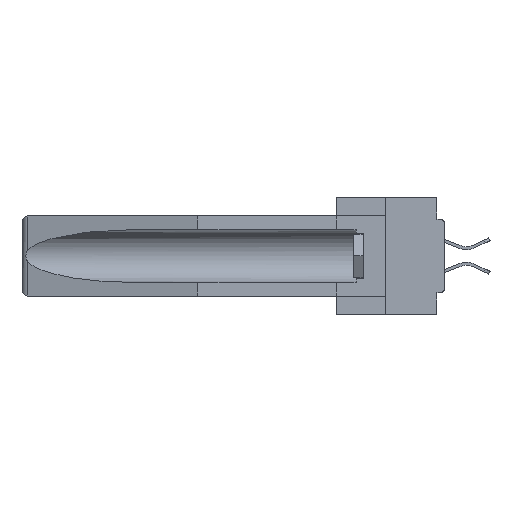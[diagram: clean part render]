
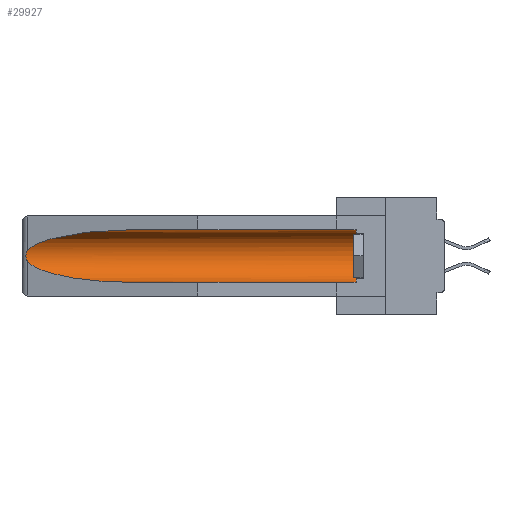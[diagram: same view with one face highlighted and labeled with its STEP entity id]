
A CAD part, left-side view. The second image highlights one B-rep face of the part: STEP entity #29927.
In plain terms, the highlighted cylindrical face has radius 2.857 mm (diameter 5.715 mm), a partial arc.
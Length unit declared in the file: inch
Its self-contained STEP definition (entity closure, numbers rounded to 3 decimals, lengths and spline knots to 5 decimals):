
#23 = DIRECTION ( 'NONE',  ( 0., 1., 0. ) ) ;
#1251 = CARTESIAN_POINT ( 'NONE',  ( 0.26537, 1.52718, -0.19328 ) ) ;
#2004 = CARTESIAN_POINT ( 'NONE',  ( 0.2673, 1.5327, -0.16383 ) ) ;
#4246 = AXIS2_PLACEMENT_3D ( 'NONE', #12824, #24051, #27007 ) ;
#5153 = EDGE_CURVE ( 'NONE', #10641, #20374, #31416, .T. ) ;
#5657 = CARTESIAN_POINT ( 'NONE',  ( 0.21114, 1.30732, -0.284 ) ) ;
#6368 = VERTEX_POINT ( 'NONE', #16135 ) ;
#6441 = VERTEX_POINT ( 'NONE', #9119 ) ;
#7537 = ORIENTED_EDGE ( 'NONE', *, *, #33902, .T. ) ;
#7726 = CARTESIAN_POINT ( 'NONE',  ( 0.155, 0.126, -0.059 ) ) ;
#8056 = CARTESIAN_POINT ( 'NONE',  ( 0.155, -0.30754, -0.059 ) ) ;
#9038 = ORIENTED_EDGE ( 'NONE', *, *, #23581, .T. ) ;
#9119 = CARTESIAN_POINT ( 'NONE',  ( 0.26537, 1.52718, -0.14972 ) ) ;
#9390 = CARTESIAN_POINT ( 'NONE',  ( 0.2675, 1.53308, -0.17534 ) ) ;
#10641 = VERTEX_POINT ( 'NONE', #1251 ) ;
#12159 = B_SPLINE_CURVE_WITH_KNOTS ( 'NONE', 3,
 ( #22994, #21154, #17908, #2004, #32044, #9390, #32305, #32420, #18926, #15101 ),
 .UNSPECIFIED., .F., .F.,
 ( 4, 2, 2, 2, 4 ),
 ( 0., 0.00029, 0.00058, 0.00087, 0.00117 ),
 .UNSPECIFIED. ) ;
#12186 = VERTEX_POINT ( 'NONE', #7726 ) ;
#12824 = CARTESIAN_POINT ( 'NONE',  ( 0.155, -0.30754, -0.1715 ) ) ;
#13174 = CARTESIAN_POINT ( 'NONE',  ( 0.155, 1.07973, -0.059 ) ) ;
#15101 = CARTESIAN_POINT ( 'NONE',  ( 0.26537, 1.52718, -0.19328 ) ) ;
#15527 = DIRECTION ( 'NONE',  ( 0., -1., 0. ) ) ;
#15955 = EDGE_LOOP ( 'NONE', ( #26120, #7537, #26296, #22930, #9038, #35667 ) ) ;
#16126 = CARTESIAN_POINT ( 'NONE',  ( 0.26537, 1.52718, -0.14972 ) ) ;
#16135 = CARTESIAN_POINT ( 'NONE',  ( 0.155, 1.07973, -0.059 ) ) ;
#16398 = CYLINDRICAL_SURFACE ( 'NONE', #4246, 0.1125 ) ;
#17908 = CARTESIAN_POINT ( 'NONE',  ( 0.26654, 1.53092, -0.15636 ) ) ;
#18282 =( BOUNDED_CURVE ( )  B_SPLINE_CURVE ( 3, ( #13174, #32949, #33077, #16126 ),
 .UNSPECIFIED., .F., .F. ) 
 B_SPLINE_CURVE_WITH_KNOTS ( ( 4, 4 ),
 ( 4.71239, 6.08839 ),
 .UNSPECIFIED. ) 
 CURVE ( )  GEOMETRIC_REPRESENTATION_ITEM ( )  RATIONAL_B_SPLINE_CURVE ( ( 1., 0.848, 0.848, 1. ) ) 
 REPRESENTATION_ITEM ( '' )  );
#18366 = DIRECTION ( 'NONE',  ( 0., 0., 1. ) ) ;
#18926 = CARTESIAN_POINT ( 'NONE',  ( 0.26597, 1.5296, -0.19026 ) ) ;
#19382 = EDGE_CURVE ( 'NONE', #6368, #6441, #18282, .T. ) ;
#19997 = CARTESIAN_POINT ( 'NONE',  ( 0.155, -0.30754, -0.284 ) ) ;
#20374 = VERTEX_POINT ( 'NONE', #34855 ) ;
#21154 = CARTESIAN_POINT ( 'NONE',  ( 0.26597, 1.52961, -0.15275 ) ) ;
#21763 = EDGE_CURVE ( 'NONE', #35804, #20374, #28315, .T. ) ;
#22930 = ORIENTED_EDGE ( 'NONE', *, *, #21763, .F. ) ;
#22994 = CARTESIAN_POINT ( 'NONE',  ( 0.26537, 1.52718, -0.14972 ) ) ;
#23581 = EDGE_CURVE ( 'NONE', #35804, #12186, #28172, .T. ) ;
#23667 = CARTESIAN_POINT ( 'NONE',  ( 0.155, 0.126, -0.1715 ) ) ;
#23923 = FACE_OUTER_BOUND ( 'NONE', #15955, .T. ) ;
#24051 = DIRECTION ( 'NONE',  ( 0., 1., 0. ) ) ;
#24090 = EDGE_CURVE ( 'NONE', #12186, #6368, #34822, .T. ) ;
#24212 = VECTOR ( 'NONE', #23, 39.37008 ) ;
#26009 = CARTESIAN_POINT ( 'NONE',  ( 0.155, 0.126, -0.284 ) ) ;
#26055 = CARTESIAN_POINT ( 'NONE',  ( 0.26537, 1.52718, -0.19328 ) ) ;
#26120 = ORIENTED_EDGE ( 'NONE', *, *, #19382, .T. ) ;
#26296 = ORIENTED_EDGE ( 'NONE', *, *, #5153, .T. ) ;
#27007 = DIRECTION ( 'NONE',  ( 0., 0., 1. ) ) ;
#28172 = CIRCLE ( 'NONE', #32915, 0.1125 ) ;
#28315 = LINE ( 'NONE', #19997, #31399 ) ;
#28421 = DIRECTION ( 'NONE',  ( 0., 1., 0. ) ) ;
#29927 = ADVANCED_FACE ( 'NONE', ( #23923 ), #16398, .F. ) ;
#31399 = VECTOR ( 'NONE', #28421, 39.37008 ) ;
#31416 =( BOUNDED_CURVE ( )  B_SPLINE_CURVE ( 3, ( #26055, #33853, #5657, #36429 ),
 .UNSPECIFIED., .F., .F. ) 
 B_SPLINE_CURVE_WITH_KNOTS ( ( 4, 4 ),
 ( 0.1948, 1.5708 ),
 .UNSPECIFIED. ) 
 CURVE ( )  GEOMETRIC_REPRESENTATION_ITEM ( )  RATIONAL_B_SPLINE_CURVE ( ( 1., 0.848, 0.848, 1. ) ) 
 REPRESENTATION_ITEM ( '' )  );
#32044 = CARTESIAN_POINT ( 'NONE',  ( 0.2675, 1.53308, -0.16763 ) ) ;
#32305 = CARTESIAN_POINT ( 'NONE',  ( 0.2673, 1.53269, -0.17917 ) ) ;
#32420 = CARTESIAN_POINT ( 'NONE',  ( 0.26655, 1.53094, -0.18657 ) ) ;
#32915 = AXIS2_PLACEMENT_3D ( 'NONE', #23667, #15527, #18366 ) ;
#32949 = CARTESIAN_POINT ( 'NONE',  ( 0.21114, 1.30732, -0.059 ) ) ;
#33077 = CARTESIAN_POINT ( 'NONE',  ( 0.25451, 1.48313, -0.09465 ) ) ;
#33853 = CARTESIAN_POINT ( 'NONE',  ( 0.25451, 1.48313, -0.24835 ) ) ;
#33902 = EDGE_CURVE ( 'NONE', #6441, #10641, #12159, .T. ) ;
#34822 = LINE ( 'NONE', #8056, #24212 ) ;
#34855 = CARTESIAN_POINT ( 'NONE',  ( 0.155, 1.07973, -0.284 ) ) ;
#35667 = ORIENTED_EDGE ( 'NONE', *, *, #24090, .T. ) ;
#35804 = VERTEX_POINT ( 'NONE', #26009 ) ;
#36429 = CARTESIAN_POINT ( 'NONE',  ( 0.155, 1.07973, -0.284 ) ) ;
